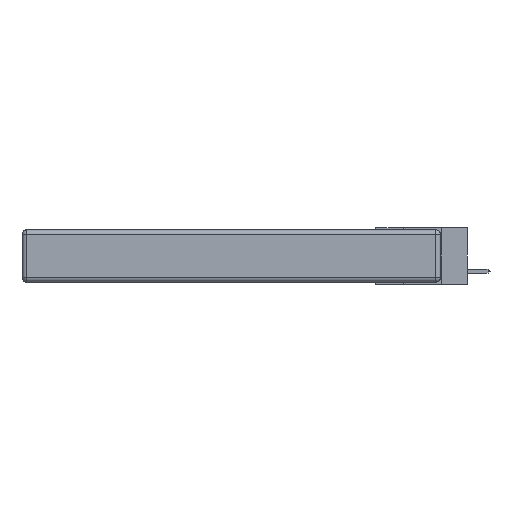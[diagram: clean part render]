
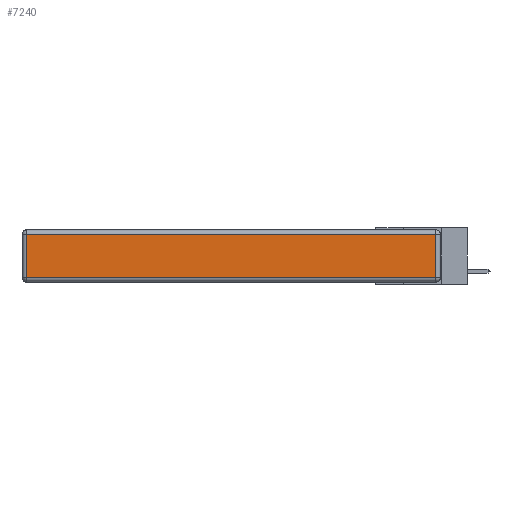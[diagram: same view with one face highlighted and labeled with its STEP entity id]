
A CAD part, left-side view. The second image highlights one B-rep face of the part: STEP entity #7240.
In plain terms, the highlighted planar face has unit normal (-1, 0, 0).
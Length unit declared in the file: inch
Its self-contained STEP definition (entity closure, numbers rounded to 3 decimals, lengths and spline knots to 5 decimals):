
#838 = VECTOR ( 'NONE', #19883, 39.37008 ) ;
#1123 = DIRECTION ( 'NONE',  ( 0., 0., 1. ) ) ;
#2167 = AXIS2_PLACEMENT_3D ( 'NONE', #17015, #17124, #1123 ) ;
#2255 = CARTESIAN_POINT ( 'NONE',  ( 0., 0.03, -0.343 ) ) ;
#2819 = EDGE_CURVE ( 'NONE', #14060, #5275, #10808, .T. ) ;
#4448 = CARTESIAN_POINT ( 'NONE',  ( 0., 0.03, -0.03 ) ) ;
#5275 = VERTEX_POINT ( 'NONE', #4448 ) ;
#5644 = VECTOR ( 'NONE', #22917, 39.37008 ) ;
#6493 = CARTESIAN_POINT ( 'NONE',  ( 0., 0., -0.313 ) ) ;
#7240 = ADVANCED_FACE ( 'NONE', ( #15352 ), #33329, .T. ) ;
#7739 = DIRECTION ( 'NONE',  ( 0., 0., 1. ) ) ;
#10808 = LINE ( 'NONE', #2255, #31414 ) ;
#11826 = CARTESIAN_POINT ( 'NONE',  ( 0., 2.72, -0.03 ) ) ;
#14060 = VERTEX_POINT ( 'NONE', #32147 ) ;
#15352 = FACE_OUTER_BOUND ( 'NONE', #25765, .T. ) ;
#16014 = CARTESIAN_POINT ( 'NONE',  ( 0., 2.72, -0.313 ) ) ;
#16590 = EDGE_CURVE ( 'NONE', #30907, #14060, #27497, .T. ) ;
#16982 = CARTESIAN_POINT ( 'NONE',  ( 0., 2.75, -0.03 ) ) ;
#17015 = CARTESIAN_POINT ( 'NONE',  ( 0., 0., -0.343 ) ) ;
#17100 = DIRECTION ( 'NONE',  ( 0., 1., 0. ) ) ;
#17124 = DIRECTION ( 'NONE',  ( -1., 0., 0. ) ) ;
#19573 = ORIENTED_EDGE ( 'NONE', *, *, #16590, .T. ) ;
#19883 = DIRECTION ( 'NONE',  ( 0., 0., -1. ) ) ;
#21491 = EDGE_CURVE ( 'NONE', #5275, #25441, #23864, .T. ) ;
#22280 = ORIENTED_EDGE ( 'NONE', *, *, #21491, .T. ) ;
#22917 = DIRECTION ( 'NONE',  ( 0., -1., 0. ) ) ;
#23017 = VECTOR ( 'NONE', #17100, 39.37008 ) ;
#23864 = LINE ( 'NONE', #16982, #23017 ) ;
#25441 = VERTEX_POINT ( 'NONE', #11826 ) ;
#25765 = EDGE_LOOP ( 'NONE', ( #19573, #33538, #22280, #33607 ) ) ;
#27274 = LINE ( 'NONE', #30497, #838 ) ;
#27497 = LINE ( 'NONE', #6493, #5644 ) ;
#30497 = CARTESIAN_POINT ( 'NONE',  ( 0., 2.72, -0.343 ) ) ;
#30907 = VERTEX_POINT ( 'NONE', #16014 ) ;
#31414 = VECTOR ( 'NONE', #7739, 39.37008 ) ;
#32147 = CARTESIAN_POINT ( 'NONE',  ( 0., 0.03, -0.313 ) ) ;
#32565 = EDGE_CURVE ( 'NONE', #25441, #30907, #27274, .T. ) ;
#33329 = PLANE ( 'NONE',  #2167 ) ;
#33538 = ORIENTED_EDGE ( 'NONE', *, *, #2819, .T. ) ;
#33607 = ORIENTED_EDGE ( 'NONE', *, *, #32565, .T. ) ;
